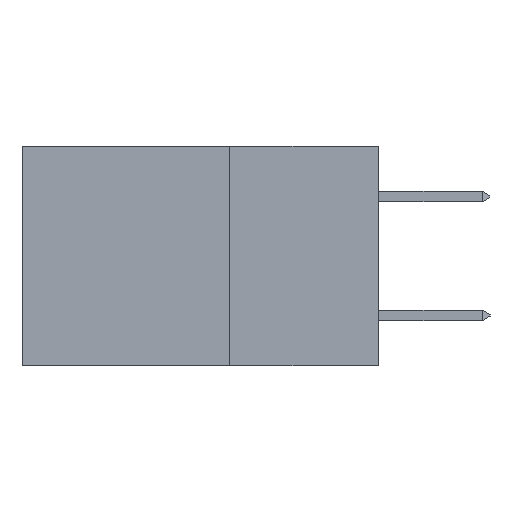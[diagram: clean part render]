
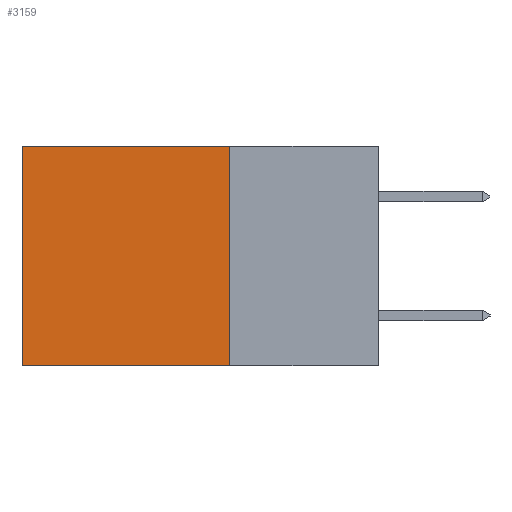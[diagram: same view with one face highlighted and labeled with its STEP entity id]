
A CAD part, left-side view. The second image highlights one B-rep face of the part: STEP entity #3159.
In plain terms, the highlighted planar face has unit normal (-1, 0, 0).
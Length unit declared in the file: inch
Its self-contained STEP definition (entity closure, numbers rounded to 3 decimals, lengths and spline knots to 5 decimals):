
#331 = LINE ( 'NONE', #18328, #15622 ) ;
#1125 = VECTOR ( 'NONE', #21553, 39.37008 ) ;
#1144 = EDGE_CURVE ( 'NONE', #4230, #3665, #7084, .T. ) ;
#2176 = VECTOR ( 'NONE', #3219, 39.37008 ) ;
#3159 = ADVANCED_FACE ( 'NONE', ( #16986 ), #10769, .F. ) ;
#3219 = DIRECTION ( 'NONE',  ( 0., 1., 0. ) ) ;
#3543 = CARTESIAN_POINT ( 'NONE',  ( 0.2615, 0.25, 0. ) ) ;
#3665 = VERTEX_POINT ( 'NONE', #5405 ) ;
#3949 = AXIS2_PLACEMENT_3D ( 'NONE', #10768, #10713, #10691 ) ;
#4230 = VERTEX_POINT ( 'NONE', #3543 ) ;
#5405 = CARTESIAN_POINT ( 'NONE',  ( 0.2615, 0.25, -0.37 ) ) ;
#7084 = LINE ( 'NONE', #21276, #1125 ) ;
#7501 = LINE ( 'NONE', #17197, #2176 ) ;
#8387 = DIRECTION ( 'NONE',  ( 0., 1., 0. ) ) ;
#9807 = CARTESIAN_POINT ( 'NONE',  ( 0.2615, 0.6, -0.37 ) ) ;
#10691 = DIRECTION ( 'NONE',  ( 0., 0., -1. ) ) ;
#10713 = DIRECTION ( 'NONE',  ( 1., 0., 0. ) ) ;
#10768 = CARTESIAN_POINT ( 'NONE',  ( 0.2615, 0.25, -0.37 ) ) ;
#10769 = PLANE ( 'NONE',  #3949 ) ;
#15422 = CARTESIAN_POINT ( 'NONE',  ( 0.2615, 0.6, 0. ) ) ;
#15622 = VECTOR ( 'NONE', #8387, 39.37008 ) ;
#16361 = CARTESIAN_POINT ( 'NONE',  ( 0.2615, 0.6, -0.37 ) ) ;
#16454 = EDGE_CURVE ( 'NONE', #3665, #19084, #7501, .T. ) ;
#16986 = FACE_OUTER_BOUND ( 'NONE', #21736, .T. ) ;
#17197 = CARTESIAN_POINT ( 'NONE',  ( 0.2615, 0.25, -0.37 ) ) ;
#17612 = LINE ( 'NONE', #16361, #22900 ) ;
#18328 = CARTESIAN_POINT ( 'NONE',  ( 0.2615, 0.25, 0. ) ) ;
#18385 = DIRECTION ( 'NONE',  ( 0., 0., -1. ) ) ;
#19084 = VERTEX_POINT ( 'NONE', #9807 ) ;
#19674 = VERTEX_POINT ( 'NONE', #15422 ) ;
#19973 = EDGE_CURVE ( 'NONE', #19674, #19084, #17612, .T. ) ;
#21276 = CARTESIAN_POINT ( 'NONE',  ( 0.2615, 0.25, -0.37 ) ) ;
#21553 = DIRECTION ( 'NONE',  ( 0., 0., -1. ) ) ;
#21736 = EDGE_LOOP ( 'NONE', ( #25195, #23264, #22427, #23507 ) ) ;
#22427 = ORIENTED_EDGE ( 'NONE', *, *, #1144, .F. ) ;
#22900 = VECTOR ( 'NONE', #18385, 39.37008 ) ;
#23016 = EDGE_CURVE ( 'NONE', #4230, #19674, #331, .T. ) ;
#23264 = ORIENTED_EDGE ( 'NONE', *, *, #16454, .F. ) ;
#23507 = ORIENTED_EDGE ( 'NONE', *, *, #23016, .T. ) ;
#25195 = ORIENTED_EDGE ( 'NONE', *, *, #19973, .T. ) ;
